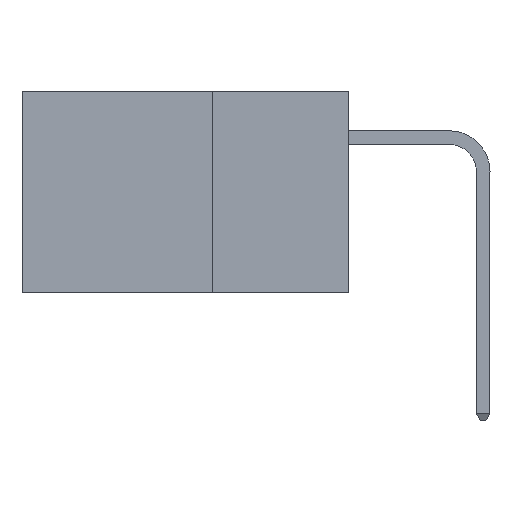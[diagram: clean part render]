
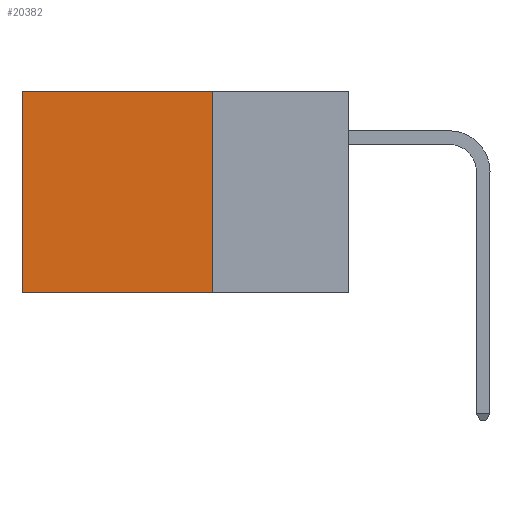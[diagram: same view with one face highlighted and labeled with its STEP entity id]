
A CAD part, left-side view. The second image highlights one B-rep face of the part: STEP entity #20382.
In plain terms, the highlighted planar face has unit normal (-1, 0, 0).
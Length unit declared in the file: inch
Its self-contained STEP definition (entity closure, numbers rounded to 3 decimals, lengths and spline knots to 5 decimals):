
#9 = ORIENTED_EDGE ( 'NONE', *, *, #7565, .F. ) ;
#1983 = DIRECTION ( 'NONE',  ( 1., 0., 0. ) ) ;
#2152 = DIRECTION ( 'NONE',  ( 0., 0., -1. ) ) ;
#2394 = DIRECTION ( 'NONE',  ( 0., 0., -1. ) ) ;
#2487 = DIRECTION ( 'NONE',  ( 0., 0., -1. ) ) ;
#3967 = DIRECTION ( 'NONE',  ( 0., 1., 0. ) ) ;
#5255 = VECTOR ( 'NONE', #2394, 39.37008 ) ;
#7565 = EDGE_CURVE ( 'NONE', #13023, #24634, #10472, .T. ) ;
#8409 = CARTESIAN_POINT ( 'NONE',  ( 0.2875, 0.6, -0.37 ) ) ;
#10472 = LINE ( 'NONE', #22291, #14707 ) ;
#10589 = DIRECTION ( 'NONE',  ( 0., 1., 0. ) ) ;
#11591 = AXIS2_PLACEMENT_3D ( 'NONE', #11783, #1983, #2152 ) ;
#11783 = CARTESIAN_POINT ( 'NONE',  ( 0.2875, 0.25, 0. ) ) ;
#11853 = EDGE_CURVE ( 'NONE', #13023, #23535, #19193, .T. ) ;
#11985 = VERTEX_POINT ( 'NONE', #8409 ) ;
#12039 = CARTESIAN_POINT ( 'NONE',  ( 0.2875, 0.25, -0.37 ) ) ;
#13023 = VERTEX_POINT ( 'NONE', #24788 ) ;
#13561 = LINE ( 'NONE', #21870, #15685 ) ;
#14707 = VECTOR ( 'NONE', #2487, 39.37008 ) ;
#15400 = ORIENTED_EDGE ( 'NONE', *, *, #15756, .T. ) ;
#15483 = LINE ( 'NONE', #21553, #5255 ) ;
#15685 = VECTOR ( 'NONE', #10589, 39.37008 ) ;
#15756 = EDGE_CURVE ( 'NONE', #23535, #11985, #15483, .T. ) ;
#16792 = VECTOR ( 'NONE', #3967, 39.37008 ) ;
#18391 = ORIENTED_EDGE ( 'NONE', *, *, #11853, .T. ) ;
#19141 = FACE_OUTER_BOUND ( 'NONE', #23359, .T. ) ;
#19193 = LINE ( 'NONE', #21385, #16792 ) ;
#20317 = ORIENTED_EDGE ( 'NONE', *, *, #23019, .F. ) ;
#20382 = ADVANCED_FACE ( 'NONE', ( #19141 ), #23333, .F. ) ;
#21385 = CARTESIAN_POINT ( 'NONE',  ( 0.2875, 0.25, 0. ) ) ;
#21553 = CARTESIAN_POINT ( 'NONE',  ( 0.2875, 0.6, 0. ) ) ;
#21870 = CARTESIAN_POINT ( 'NONE',  ( 0.2875, 0.25, -0.37 ) ) ;
#22291 = CARTESIAN_POINT ( 'NONE',  ( 0.2875, 0.25, 0. ) ) ;
#22427 = CARTESIAN_POINT ( 'NONE',  ( 0.2875, 0.6, 0. ) ) ;
#23019 = EDGE_CURVE ( 'NONE', #24634, #11985, #13561, .T. ) ;
#23333 = PLANE ( 'NONE',  #11591 ) ;
#23359 = EDGE_LOOP ( 'NONE', ( #15400, #20317, #9, #18391 ) ) ;
#23535 = VERTEX_POINT ( 'NONE', #22427 ) ;
#24634 = VERTEX_POINT ( 'NONE', #12039 ) ;
#24788 = CARTESIAN_POINT ( 'NONE',  ( 0.2875, 0.25, 0. ) ) ;
